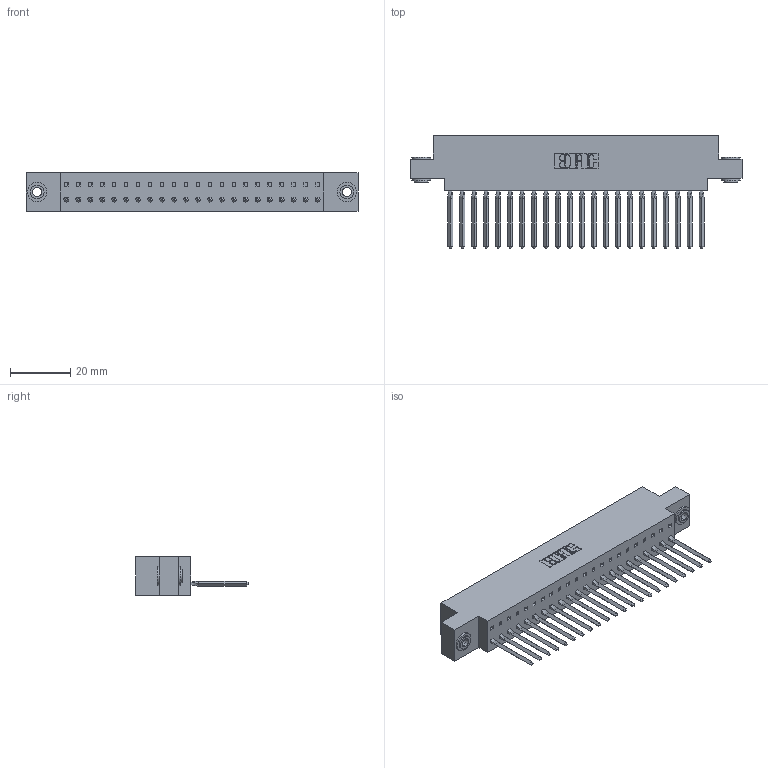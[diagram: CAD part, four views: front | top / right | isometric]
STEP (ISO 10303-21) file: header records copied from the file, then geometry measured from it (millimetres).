
FILE_DESCRIPTION (( 'STEP AP203' ), '1' );
FILE_NAME ('317-022-541-603.STEP', '2020-02-27T17:16:10', ( '' ), ( '' ), 'SwSTEP 2.0', 'SolidWorks 2016', '' );
FILE_SCHEMA (( 'CONFIG_CONTROL_DESIGN' ));
Length unit declared in the file: inch
Products named in the file (4): 317-290-002_541; 317-022-541-603; 317 Part_.156 Dia - TH; 345-250-002_345-250-002-102
Assembly tree (25 placements, depth 2):
  317-022-541-603
    317 Part_.156 Dia - TH
    317-290-002_541  x22
    345-250-002_345-250-002-102  x2
Bounding box: 109.88 x 37.34 x 12.7 mm (x, y, z)
Volume: 17223.3 mm3; surface area: 23885.6 mm2
Topology: 25 solids, 25 shells, 3484 faces, 9899 edges, 6434 vertices
Faces by surface type: plane 2796, cylinder 592, bspline 88, cone 8
Entity records: 36085 total; most frequent: CARTESIAN_POINT 7014, ORIENTED_EDGE 6282, DIRECTION 5187, EDGE_CURVE 3141, VECTOR 2753, LINE 2753, VERTEX_POINT 2084, AXIS2_PLACEMENT_3D 1217
